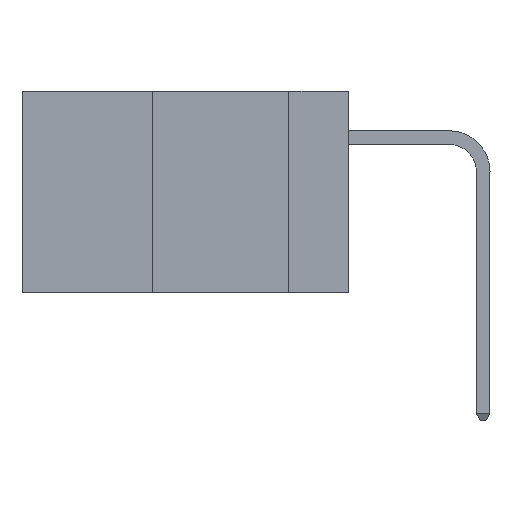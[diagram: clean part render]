
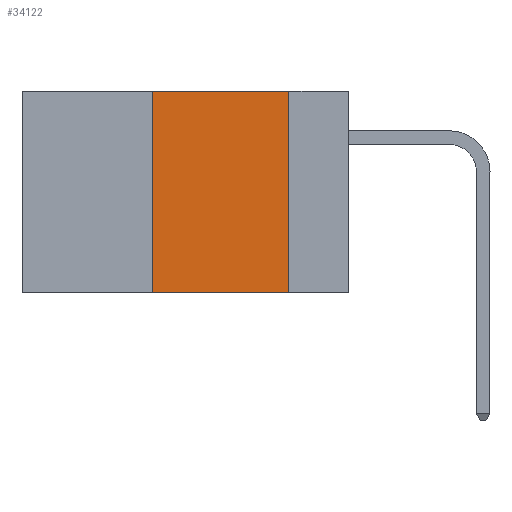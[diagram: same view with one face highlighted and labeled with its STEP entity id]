
A CAD part, left-side view. The second image highlights one B-rep face of the part: STEP entity #34122.
In plain terms, the highlighted planar face has unit normal (-1, 0, 0).
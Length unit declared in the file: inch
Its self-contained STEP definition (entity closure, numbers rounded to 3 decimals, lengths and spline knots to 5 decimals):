
#271 = ORIENTED_EDGE ( 'NONE', *, *, #17741, .F. ) ;
#885 = ORIENTED_EDGE ( 'NONE', *, *, #30366, .F. ) ;
#2418 = DIRECTION ( 'NONE',  ( 0., 0., -1. ) ) ;
#2441 = DIRECTION ( 'NONE',  ( 0., -1., 0. ) ) ;
#3149 = VERTEX_POINT ( 'NONE', #5553 ) ;
#3950 = AXIS2_PLACEMENT_3D ( 'NONE', #16576, #4132, #4413 ) ;
#4132 = DIRECTION ( 'NONE',  ( 1., 0., 0. ) ) ;
#4413 = DIRECTION ( 'NONE',  ( 0., 0., -1. ) ) ;
#5349 = EDGE_LOOP ( 'NONE', ( #18404, #885, #271, #10387 ) ) ;
#5553 = CARTESIAN_POINT ( 'NONE',  ( 0., 0.11, -0.37 ) ) ;
#9338 = CARTESIAN_POINT ( 'NONE',  ( 0., 0.11, 0. ) ) ;
#10387 = ORIENTED_EDGE ( 'NONE', *, *, #36850, .T. ) ;
#12233 = LINE ( 'NONE', #35689, #35466 ) ;
#12618 = VERTEX_POINT ( 'NONE', #9338 ) ;
#12855 = VECTOR ( 'NONE', #31812, 39.37008 ) ;
#12930 = LINE ( 'NONE', #19179, #33293 ) ;
#14219 = EDGE_CURVE ( 'NONE', #12618, #3149, #22474, .T. ) ;
#16199 = VERTEX_POINT ( 'NONE', #36416 ) ;
#16576 = CARTESIAN_POINT ( 'NONE',  ( 0., 0.6, 0. ) ) ;
#17741 = EDGE_CURVE ( 'NONE', #25986, #16199, #12930, .T. ) ;
#18404 = ORIENTED_EDGE ( 'NONE', *, *, #14219, .F. ) ;
#18632 = FACE_OUTER_BOUND ( 'NONE', #5349, .T. ) ;
#18841 = PLANE ( 'NONE',  #3950 ) ;
#19179 = CARTESIAN_POINT ( 'NONE',  ( 0., 0.36, 0. ) ) ;
#21239 = CARTESIAN_POINT ( 'NONE',  ( 0., 0.36, -0.37 ) ) ;
#22474 = LINE ( 'NONE', #23974, #25288 ) ;
#23974 = CARTESIAN_POINT ( 'NONE',  ( 0., 0.11, 0. ) ) ;
#25288 = VECTOR ( 'NONE', #2418, 39.37008 ) ;
#25723 = CARTESIAN_POINT ( 'NONE',  ( 0., 0.6, 0. ) ) ;
#25986 = VERTEX_POINT ( 'NONE', #21239 ) ;
#30366 = EDGE_CURVE ( 'NONE', #16199, #12618, #38496, .T. ) ;
#31812 = DIRECTION ( 'NONE',  ( 0., -1., 0. ) ) ;
#33293 = VECTOR ( 'NONE', #34487, 39.37008 ) ;
#34122 = ADVANCED_FACE ( 'NONE', ( #18632 ), #18841, .F. ) ;
#34487 = DIRECTION ( 'NONE',  ( 0., 0., 1. ) ) ;
#35466 = VECTOR ( 'NONE', #2441, 39.37008 ) ;
#35689 = CARTESIAN_POINT ( 'NONE',  ( 0., 0.6, -0.37 ) ) ;
#36416 = CARTESIAN_POINT ( 'NONE',  ( 0., 0.36, 0. ) ) ;
#36850 = EDGE_CURVE ( 'NONE', #25986, #3149, #12233, .T. ) ;
#38496 = LINE ( 'NONE', #25723, #12855 ) ;
